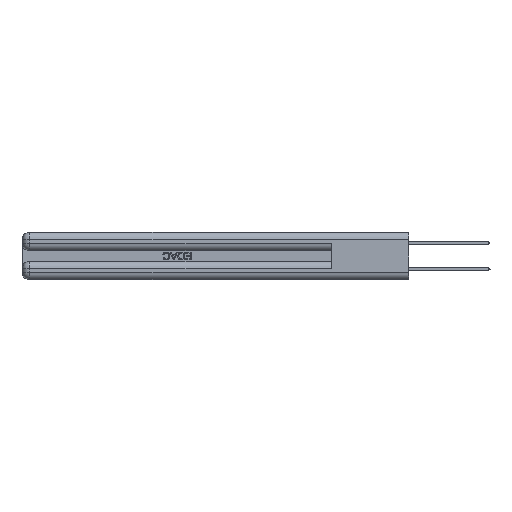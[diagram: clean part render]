
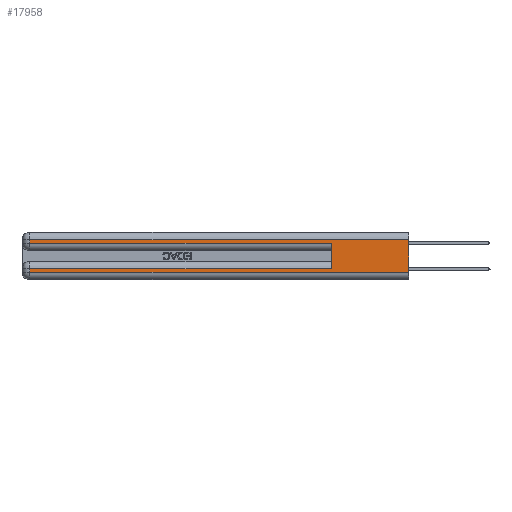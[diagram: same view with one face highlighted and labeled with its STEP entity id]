
A CAD part, left-side view. The second image highlights one B-rep face of the part: STEP entity #17958.
In plain terms, the highlighted planar face has unit normal (-1, 0, 0).
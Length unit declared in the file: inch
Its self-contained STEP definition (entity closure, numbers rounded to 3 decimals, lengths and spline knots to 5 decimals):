
#612 = VERTEX_POINT ( 'NONE', #24210 ) ;
#844 = CARTESIAN_POINT ( 'NONE',  ( 0., 0., 0.06 ) ) ;
#3524 = EDGE_CURVE ( 'NONE', #47240, #42485, #44154, .T. ) ;
#4667 = EDGE_CURVE ( 'NONE', #10996, #47240, #44020, .T. ) ;
#5334 = DIRECTION ( 'NONE',  ( 0., 0., -1. ) ) ;
#6383 = ORIENTED_EDGE ( 'NONE', *, *, #42140, .T. ) ;
#6934 = VECTOR ( 'NONE', #30653, 39.37008 ) ;
#8029 = DIRECTION ( 'NONE',  ( 0., 0., 1. ) ) ;
#9435 = LINE ( 'NONE', #9593, #33887 ) ;
#9585 = EDGE_CURVE ( 'NONE', #31789, #612, #16071, .T. ) ;
#9593 = CARTESIAN_POINT ( 'NONE',  ( 0., 0., 0.285 ) ) ;
#10996 = VERTEX_POINT ( 'NONE', #30570 ) ;
#12358 = CARTESIAN_POINT ( 'NONE',  ( 0., 2.94, 0.37 ) ) ;
#12658 = DIRECTION ( 'NONE',  ( 0., 1., 0. ) ) ;
#13207 = VERTEX_POINT ( 'NONE', #24614 ) ;
#14662 = DIRECTION ( 'NONE',  ( 0., 0., -1. ) ) ;
#15380 = CARTESIAN_POINT ( 'NONE',  ( 0., 0.6, 0.145 ) ) ;
#16071 = LINE ( 'NONE', #844, #6934 ) ;
#16945 = DIRECTION ( 'NONE',  ( 0., -1., 0. ) ) ;
#17958 = ADVANCED_FACE ( 'NONE', ( #28392 ), #43830, .F. ) ;
#17979 = VECTOR ( 'NONE', #26907, 39.37008 ) ;
#18527 = DIRECTION ( 'NONE',  ( 1., 0., 0. ) ) ;
#18977 = EDGE_CURVE ( 'NONE', #31644, #31789, #27719, .T. ) ;
#19179 = CARTESIAN_POINT ( 'NONE',  ( 0., 2.94, 0.285 ) ) ;
#20594 = ORIENTED_EDGE ( 'NONE', *, *, #18977, .T. ) ;
#22049 = ORIENTED_EDGE ( 'NONE', *, *, #4667, .T. ) ;
#22488 = ORIENTED_EDGE ( 'NONE', *, *, #3524, .T. ) ;
#22964 = LINE ( 'NONE', #46347, #45820 ) ;
#23099 = CARTESIAN_POINT ( 'NONE',  ( 0., 2.94, 0.37 ) ) ;
#23529 = CARTESIAN_POINT ( 'NONE',  ( 0., 2.94, 0.085 ) ) ;
#24210 = CARTESIAN_POINT ( 'NONE',  ( 0., 0., 0.06 ) ) ;
#24614 = CARTESIAN_POINT ( 'NONE',  ( 0., 0.6, 0.285 ) ) ;
#24736 = VECTOR ( 'NONE', #12658, 39.37008 ) ;
#25875 = DIRECTION ( 'NONE',  ( 0., 0., -1. ) ) ;
#26907 = DIRECTION ( 'NONE',  ( 0., 0., -1. ) ) ;
#27291 = CARTESIAN_POINT ( 'NONE',  ( 0., 0.6, 0.085 ) ) ;
#27719 = LINE ( 'NONE', #12358, #17979 ) ;
#28392 = FACE_OUTER_BOUND ( 'NONE', #30132, .T. ) ;
#30132 = EDGE_LOOP ( 'NONE', ( #42951, #22049, #22488, #38465, #30625, #6383, #20594, #33708 ) ) ;
#30570 = CARTESIAN_POINT ( 'NONE',  ( 0., 0., 0.31 ) ) ;
#30625 = ORIENTED_EDGE ( 'NONE', *, *, #45159, .F. ) ;
#30653 = DIRECTION ( 'NONE',  ( 0., -1., 0. ) ) ;
#31644 = VERTEX_POINT ( 'NONE', #23529 ) ;
#31789 = VERTEX_POINT ( 'NONE', #46488 ) ;
#33708 = ORIENTED_EDGE ( 'NONE', *, *, #9585, .T. ) ;
#33887 = VECTOR ( 'NONE', #16945, 39.37008 ) ;
#34155 = CARTESIAN_POINT ( 'NONE',  ( 0., 0., 0.31 ) ) ;
#34511 = VECTOR ( 'NONE', #14662, 39.37008 ) ;
#35997 = EDGE_CURVE ( 'NONE', #42485, #13207, #9435, .T. ) ;
#36426 = LINE ( 'NONE', #38177, #44996 ) ;
#38177 = CARTESIAN_POINT ( 'NONE',  ( 0., 0., 0.37 ) ) ;
#38465 = ORIENTED_EDGE ( 'NONE', *, *, #35997, .T. ) ;
#38655 = VERTEX_POINT ( 'NONE', #27291 ) ;
#40913 = CARTESIAN_POINT ( 'NONE',  ( 0., 0., 0.37 ) ) ;
#41410 = VECTOR ( 'NONE', #8029, 39.37008 ) ;
#42140 = EDGE_CURVE ( 'NONE', #38655, #31644, #22964, .T. ) ;
#42485 = VERTEX_POINT ( 'NONE', #19179 ) ;
#42774 = DIRECTION ( 'NONE',  ( 0., 1., 0. ) ) ;
#42951 = ORIENTED_EDGE ( 'NONE', *, *, #43942, .F. ) ;
#43117 = LINE ( 'NONE', #15380, #41410 ) ;
#43355 = AXIS2_PLACEMENT_3D ( 'NONE', #40913, #18527, #25875 ) ;
#43830 = PLANE ( 'NONE',  #43355 ) ;
#43942 = EDGE_CURVE ( 'NONE', #10996, #612, #36426, .T. ) ;
#44020 = LINE ( 'NONE', #34155, #24736 ) ;
#44154 = LINE ( 'NONE', #23099, #34511 ) ;
#44852 = CARTESIAN_POINT ( 'NONE',  ( 0., 2.94, 0.31 ) ) ;
#44996 = VECTOR ( 'NONE', #5334, 39.37008 ) ;
#45159 = EDGE_CURVE ( 'NONE', #38655, #13207, #43117, .T. ) ;
#45820 = VECTOR ( 'NONE', #42774, 39.37008 ) ;
#46347 = CARTESIAN_POINT ( 'NONE',  ( 0., 0., 0.085 ) ) ;
#46488 = CARTESIAN_POINT ( 'NONE',  ( 0., 2.94, 0.06 ) ) ;
#47240 = VERTEX_POINT ( 'NONE', #44852 ) ;
